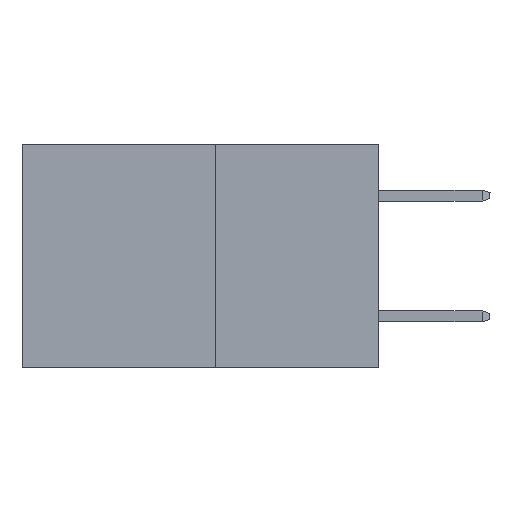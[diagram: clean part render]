
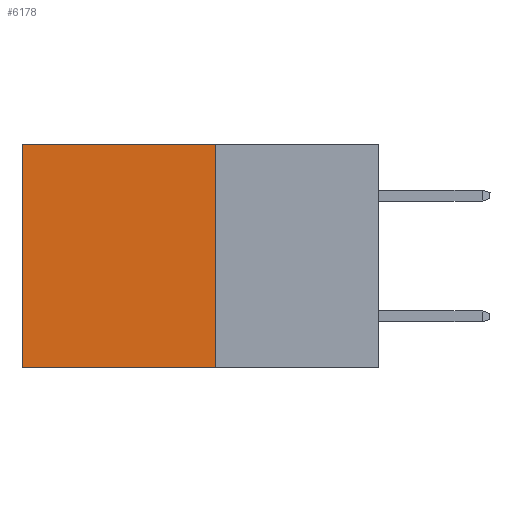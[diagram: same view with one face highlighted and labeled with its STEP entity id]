
A CAD part, left-side view. The second image highlights one B-rep face of the part: STEP entity #6178.
In plain terms, the highlighted planar face has unit normal (-1, 0, 0).
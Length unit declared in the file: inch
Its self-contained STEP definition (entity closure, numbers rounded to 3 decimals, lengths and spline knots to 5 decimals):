
#288 = CARTESIAN_POINT ( 'NONE',  ( 0.277, 0.59, -0.37 ) ) ;
#1120 = DIRECTION ( 'NONE',  ( 0., 0., -1. ) ) ;
#1264 = EDGE_CURVE ( 'NONE', #5531, #2396, #8280, .T. ) ;
#1419 = ORIENTED_EDGE ( 'NONE', *, *, #1264, .F. ) ;
#2396 = VERTEX_POINT ( 'NONE', #2558 ) ;
#2558 = CARTESIAN_POINT ( 'NONE',  ( 0.277, 0.27, -0.37 ) ) ;
#3063 = CARTESIAN_POINT ( 'NONE',  ( 0.277, 0.27, 0. ) ) ;
#3717 = CARTESIAN_POINT ( 'NONE',  ( 0.277, 0.27, 0. ) ) ;
#3892 = CARTESIAN_POINT ( 'NONE',  ( 0.277, 0.59, -0.37 ) ) ;
#3901 = LINE ( 'NONE', #288, #7822 ) ;
#4086 = LINE ( 'NONE', #9243, #5892 ) ;
#4293 = ORIENTED_EDGE ( 'NONE', *, *, #6823, .F. ) ;
#4329 = VECTOR ( 'NONE', #9848, 39.37008 ) ;
#4561 = LINE ( 'NONE', #3717, #4329 ) ;
#4676 = EDGE_LOOP ( 'NONE', ( #9519, #4293, #1419, #6343 ) ) ;
#4703 = DIRECTION ( 'NONE',  ( 1., 0., 0. ) ) ;
#5295 = FACE_OUTER_BOUND ( 'NONE', #4676, .T. ) ;
#5421 = EDGE_CURVE ( 'NONE', #5531, #9268, #4561, .T. ) ;
#5531 = VERTEX_POINT ( 'NONE', #3063 ) ;
#5594 = DIRECTION ( 'NONE',  ( 0., 0., -1. ) ) ;
#5796 = CARTESIAN_POINT ( 'NONE',  ( 0.277, 0.59, 0. ) ) ;
#5892 = VECTOR ( 'NONE', #9966, 39.37008 ) ;
#6153 = AXIS2_PLACEMENT_3D ( 'NONE', #7064, #4703, #10028 ) ;
#6178 = ADVANCED_FACE ( 'NONE', ( #5295 ), #9317, .F. ) ;
#6343 = ORIENTED_EDGE ( 'NONE', *, *, #5421, .T. ) ;
#6823 = EDGE_CURVE ( 'NONE', #2396, #8159, #4086, .T. ) ;
#7064 = CARTESIAN_POINT ( 'NONE',  ( 0.277, 0.27, -0.37 ) ) ;
#7822 = VECTOR ( 'NONE', #1120, 39.37008 ) ;
#8159 = VERTEX_POINT ( 'NONE', #3892 ) ;
#8280 = LINE ( 'NONE', #8812, #9772 ) ;
#8812 = CARTESIAN_POINT ( 'NONE',  ( 0.277, 0.27, -0.37 ) ) ;
#9243 = CARTESIAN_POINT ( 'NONE',  ( 0.277, 0.27, -0.37 ) ) ;
#9268 = VERTEX_POINT ( 'NONE', #5796 ) ;
#9317 = PLANE ( 'NONE',  #6153 ) ;
#9519 = ORIENTED_EDGE ( 'NONE', *, *, #9886, .T. ) ;
#9772 = VECTOR ( 'NONE', #5594, 39.37008 ) ;
#9848 = DIRECTION ( 'NONE',  ( 0., 1., 0. ) ) ;
#9886 = EDGE_CURVE ( 'NONE', #9268, #8159, #3901, .T. ) ;
#9966 = DIRECTION ( 'NONE',  ( 0., 1., 0. ) ) ;
#10028 = DIRECTION ( 'NONE',  ( 0., 0., -1. ) ) ;
